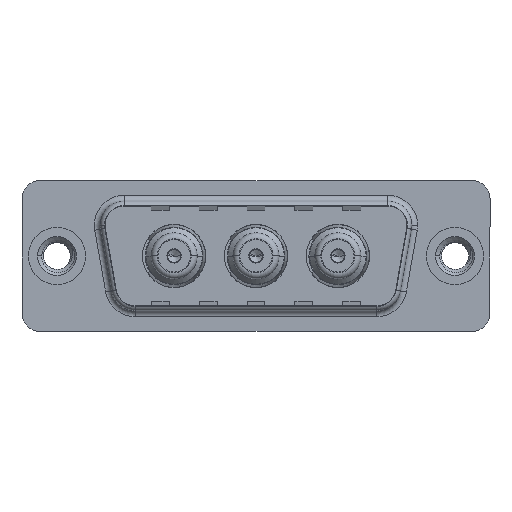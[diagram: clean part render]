
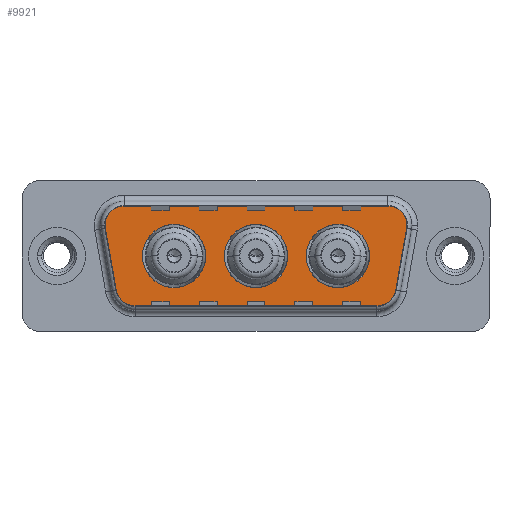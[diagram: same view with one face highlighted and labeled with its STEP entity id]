
A CAD part, top view. The second image highlights one B-rep face of the part: STEP entity #9921.
In plain terms, the highlighted planar face has unit normal (0, 0, 1).
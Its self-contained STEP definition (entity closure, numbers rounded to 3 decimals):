
#51 = AXIS2_PLACEMENT_3D ( 'NONE', #15187, #3515, #979 ) ;
#239 = CARTESIAN_POINT ( 'NONE',  ( 6.434, -4.9, 0. ) ) ;
#251 = CARTESIAN_POINT ( 'NONE',  ( 6.434, -2.9, 0. ) ) ;
#691 = DIRECTION ( 'NONE',  ( 1., 0., 0. ) ) ;
#857 = ORIENTED_EDGE ( 'NONE', *, *, #10667, .T. ) ;
#867 = AXIS2_PLACEMENT_3D ( 'NONE', #5519, #5506, #5467 ) ;
#979 = DIRECTION ( 'NONE',  ( 1., 0., 0. ) ) ;
#1030 = VERTEX_POINT ( 'NONE', #7917 ) ;
#1298 = VERTEX_POINT ( 'NONE', #6829 ) ;
#1299 = VECTOR ( 'NONE', #8191, 1000. ) ;
#1315 = CARTESIAN_POINT ( 'NONE',  ( 9.8, 0., 0. ) ) ;
#1330 = ORIENTED_EDGE ( 'NONE', *, *, #14059, .T. ) ;
#1443 = EDGE_CURVE ( 'NONE', #1030, #4064, #10518, .T. ) ;
#1541 = DIRECTION ( 'NONE',  ( -1., 0., 0. ) ) ;
#1592 = ORIENTED_EDGE ( 'NONE', *, *, #2460, .F. ) ;
#1891 = VECTOR ( 'NONE', #6079, 1000. ) ;
#2185 = EDGE_CURVE ( 'NONE', #12887, #12869, #9410, .T. ) ;
#2379 = ORIENTED_EDGE ( 'NONE', *, *, #4119, .F. ) ;
#2460 = EDGE_CURVE ( 'NONE', #14298, #6539, #10311, .T. ) ;
#2560 = ORIENTED_EDGE ( 'NONE', *, *, #7721, .T. ) ;
#2573 = CARTESIAN_POINT ( 'NONE',  ( 14., 0., 0. ) ) ;
#2613 = DIRECTION ( 'NONE',  ( 1., 0., 0. ) ) ;
#2682 = DIRECTION ( 'NONE',  ( 0., 0., 1. ) ) ;
#2700 = CARTESIAN_POINT ( 'NONE',  ( 9.8, 0., 0. ) ) ;
#3147 = ORIENTED_EDGE ( 'NONE', *, *, #7641, .F. ) ;
#3245 = FACE_BOUND ( 'NONE', #14101, .T. ) ;
#3515 = DIRECTION ( 'NONE',  ( 0., 0., 1. ) ) ;
#3645 = FACE_OUTER_BOUND ( 'NONE', #7032, .T. ) ;
#3805 = CARTESIAN_POINT ( 'NONE',  ( 29.859, 2.553, 0. ) ) ;
#3901 = AXIS2_PLACEMENT_3D ( 'NONE', #13039, #6721, #12430 ) ;
#4064 = VERTEX_POINT ( 'NONE', #6972 ) ;
#4119 = EDGE_CURVE ( 'NONE', #12869, #12887, #12084, .T. ) ;
#4198 = CARTESIAN_POINT ( 'NONE',  ( 23.5, 0., 0. ) ) ;
#4203 = AXIS2_PLACEMENT_3D ( 'NONE', #4198, #4228, #7269 ) ;
#4228 = DIRECTION ( 'NONE',  ( 0., 0., 1. ) ) ;
#4251 = CIRCLE ( 'NONE', #6933, 2.65 ) ;
#4311 = ORIENTED_EDGE ( 'NONE', *, *, #7768, .T. ) ;
#4325 = VERTEX_POINT ( 'NONE', #15284 ) ;
#4362 = CIRCLE ( 'NONE', #8724, 2. ) ;
#4693 = EDGE_LOOP ( 'NONE', ( #1592, #3147 ) ) ;
#4837 = VERTEX_POINT ( 'NONE', #14618 ) ;
#4925 = EDGE_CURVE ( 'NONE', #13434, #6711, #12734, .T. ) ;
#5047 = AXIS2_PLACEMENT_3D ( 'NONE', #2700, #2682, #2613 ) ;
#5115 = CARTESIAN_POINT ( 'NONE',  ( 5.411, 4.9, 0. ) ) ;
#5147 = DIRECTION ( 'NONE',  ( 0., 0., 1. ) ) ;
#5467 = DIRECTION ( 'NONE',  ( -1., 0., 0. ) ) ;
#5506 = DIRECTION ( 'NONE',  ( 0., 0., 1. ) ) ;
#5519 = CARTESIAN_POINT ( 'NONE',  ( 27.889, 2.9, 0. ) ) ;
#5722 = AXIS2_PLACEMENT_3D ( 'NONE', #1315, #13981, #12840 ) ;
#5753 = ORIENTED_EDGE ( 'NONE', *, *, #4925, .F. ) ;
#6059 = FACE_BOUND ( 'NONE', #13395, .T. ) ;
#6079 = DIRECTION ( 'NONE',  ( 0.174, -0.985, 0. ) ) ;
#6210 = CARTESIAN_POINT ( 'NONE',  ( 3.441, 2.553, 0. ) ) ;
#6539 = VERTEX_POINT ( 'NONE', #2573 ) ;
#6711 = VERTEX_POINT ( 'NONE', #10479 ) ;
#6721 = DIRECTION ( 'NONE',  ( 0., 0., 1. ) ) ;
#6774 = CARTESIAN_POINT ( 'NONE',  ( 26.866, -4.9, 0. ) ) ;
#6829 = CARTESIAN_POINT ( 'NONE',  ( 4.464, -3.247, 0. ) ) ;
#6839 = CARTESIAN_POINT ( 'NONE',  ( 6.434, -4.9, 0. ) ) ;
#6933 = AXIS2_PLACEMENT_3D ( 'NONE', #8994, #8979, #8976 ) ;
#6965 = DIRECTION ( 'NONE',  ( 0., 0., 1. ) ) ;
#6972 = CARTESIAN_POINT ( 'NONE',  ( 29.859, 2.553, 0. ) ) ;
#6994 = VERTEX_POINT ( 'NONE', #239 ) ;
#7032 = EDGE_LOOP ( 'NONE', ( #9422, #7982, #857, #4311, #2560, #7051, #8170, #1330, #14146 ) ) ;
#7051 = ORIENTED_EDGE ( 'NONE', *, *, #11951, .T. ) ;
#7088 = PLANE ( 'NONE',  #51 ) ;
#7269 = DIRECTION ( 'NONE',  ( 1., 0., 0. ) ) ;
#7291 = DIRECTION ( 'NONE',  ( -1., 0., 0. ) ) ;
#7641 = EDGE_CURVE ( 'NONE', #6539, #14298, #4251, .T. ) ;
#7698 = CARTESIAN_POINT ( 'NONE',  ( 12.45, 0., 0. ) ) ;
#7721 = EDGE_CURVE ( 'NONE', #11137, #8484, #11446, .T. ) ;
#7747 = EDGE_CURVE ( 'NONE', #4837, #1298, #13741, .T. ) ;
#7761 = CARTESIAN_POINT ( 'NONE',  ( 5.411, 4.9, 0. ) ) ;
#7768 = EDGE_CURVE ( 'NONE', #4325, #11137, #11098, .T. ) ;
#7917 = CARTESIAN_POINT ( 'NONE',  ( 28.836, -3.247, 0. ) ) ;
#7918 = EDGE_CURVE ( 'NONE', #6711, #13434, #8863, .T. ) ;
#7925 = CARTESIAN_POINT ( 'NONE',  ( 19.3, 0., 0. ) ) ;
#7969 = DIRECTION ( 'NONE',  ( 0., 0., 1. ) ) ;
#7982 = ORIENTED_EDGE ( 'NONE', *, *, #1443, .T. ) ;
#8026 = CIRCLE ( 'NONE', #13514, 2. ) ;
#8170 = ORIENTED_EDGE ( 'NONE', *, *, #7747, .T. ) ;
#8191 = DIRECTION ( 'NONE',  ( 0.174, 0.985, 0. ) ) ;
#8228 = LINE ( 'NONE', #6839, #11396 ) ;
#8240 = CARTESIAN_POINT ( 'NONE',  ( 27.889, 4.9, 0. ) ) ;
#8484 = VERTEX_POINT ( 'NONE', #5115 ) ;
#8724 = AXIS2_PLACEMENT_3D ( 'NONE', #13899, #6965, #15067 ) ;
#8760 = DIRECTION ( 'NONE',  ( 0., 0., 1. ) ) ;
#8775 = VERTEX_POINT ( 'NONE', #6774 ) ;
#8863 = CIRCLE ( 'NONE', #5047, 2.65 ) ;
#8976 = DIRECTION ( 'NONE',  ( 1., 0., 0. ) ) ;
#8979 = DIRECTION ( 'NONE',  ( 0., 0., 1. ) ) ;
#8994 = CARTESIAN_POINT ( 'NONE',  ( 16.65, 0., 0. ) ) ;
#9410 = CIRCLE ( 'NONE', #3901, 2.65 ) ;
#9422 = ORIENTED_EDGE ( 'NONE', *, *, #10364, .T. ) ;
#9763 = EDGE_CURVE ( 'NONE', #6994, #8775, #8228, .T. ) ;
#9921 = ADVANCED_FACE ( 'NONE', ( #12276, #6059, #3245, #3645 ), #7088, .T. ) ;
#10024 = AXIS2_PLACEMENT_3D ( 'NONE', #12161, #5147, #13306 ) ;
#10311 = CIRCLE ( 'NONE', #13312, 2.65 ) ;
#10364 = EDGE_CURVE ( 'NONE', #8775, #1030, #4362, .T. ) ;
#10479 = CARTESIAN_POINT ( 'NONE',  ( 7.15, 0., 0. ) ) ;
#10518 = LINE ( 'NONE', #3805, #1299 ) ;
#10667 = EDGE_CURVE ( 'NONE', #4064, #4325, #13135, .T. ) ;
#10830 = ORIENTED_EDGE ( 'NONE', *, *, #7918, .F. ) ;
#11098 = CIRCLE ( 'NONE', #867, 2. ) ;
#11137 = VERTEX_POINT ( 'NONE', #8240 ) ;
#11396 = VECTOR ( 'NONE', #14935, 1000. ) ;
#11446 = LINE ( 'NONE', #7761, #14109 ) ;
#11951 = EDGE_CURVE ( 'NONE', #8484, #4837, #13353, .T. ) ;
#11966 = DIRECTION ( 'NONE',  ( 0., 0., 1. ) ) ;
#12084 = CIRCLE ( 'NONE', #4203, 2.65 ) ;
#12161 = CARTESIAN_POINT ( 'NONE',  ( 27.889, 2.9, 0. ) ) ;
#12276 = FACE_BOUND ( 'NONE', #4693, .T. ) ;
#12430 = DIRECTION ( 'NONE',  ( 1., 0., 0. ) ) ;
#12730 = CARTESIAN_POINT ( 'NONE',  ( 16.65, 0., 0. ) ) ;
#12734 = CIRCLE ( 'NONE', #5722, 2.65 ) ;
#12840 = DIRECTION ( 'NONE',  ( 1., 0., 0. ) ) ;
#12869 = VERTEX_POINT ( 'NONE', #15197 ) ;
#12887 = VERTEX_POINT ( 'NONE', #14044 ) ;
#13039 = CARTESIAN_POINT ( 'NONE',  ( 23.5, 0., 0. ) ) ;
#13135 = CIRCLE ( 'NONE', #10024, 2. ) ;
#13306 = DIRECTION ( 'NONE',  ( -1., 0., 0. ) ) ;
#13312 = AXIS2_PLACEMENT_3D ( 'NONE', #12730, #11966, #13897 ) ;
#13353 = CIRCLE ( 'NONE', #13970, 2. ) ;
#13395 = EDGE_LOOP ( 'NONE', ( #2379, #14256 ) ) ;
#13434 = VERTEX_POINT ( 'NONE', #7698 ) ;
#13514 = AXIS2_PLACEMENT_3D ( 'NONE', #251, #8760, #1541 ) ;
#13741 = LINE ( 'NONE', #6210, #1891 ) ;
#13897 = DIRECTION ( 'NONE',  ( 1., 0., 0. ) ) ;
#13899 = CARTESIAN_POINT ( 'NONE',  ( 26.866, -2.9, 0. ) ) ;
#13970 = AXIS2_PLACEMENT_3D ( 'NONE', #14915, #7969, #691 ) ;
#13981 = DIRECTION ( 'NONE',  ( 0., 0., 1. ) ) ;
#14044 = CARTESIAN_POINT ( 'NONE',  ( 20.85, 0., 0. ) ) ;
#14059 = EDGE_CURVE ( 'NONE', #1298, #6994, #8026, .T. ) ;
#14101 = EDGE_LOOP ( 'NONE', ( #5753, #10830 ) ) ;
#14109 = VECTOR ( 'NONE', #7291, 1000. ) ;
#14146 = ORIENTED_EDGE ( 'NONE', *, *, #9763, .T. ) ;
#14256 = ORIENTED_EDGE ( 'NONE', *, *, #2185, .F. ) ;
#14298 = VERTEX_POINT ( 'NONE', #7925 ) ;
#14618 = CARTESIAN_POINT ( 'NONE',  ( 3.441, 2.553, 0. ) ) ;
#14915 = CARTESIAN_POINT ( 'NONE',  ( 5.411, 2.9, 0. ) ) ;
#14935 = DIRECTION ( 'NONE',  ( 1., 0., 0. ) ) ;
#15067 = DIRECTION ( 'NONE',  ( 1., 0., 0. ) ) ;
#15187 = CARTESIAN_POINT ( 'NONE',  ( 26.866, -2.9, 0. ) ) ;
#15197 = CARTESIAN_POINT ( 'NONE',  ( 26.15, 0., 0. ) ) ;
#15284 = CARTESIAN_POINT ( 'NONE',  ( 29.889, 2.9, 0. ) ) ;
